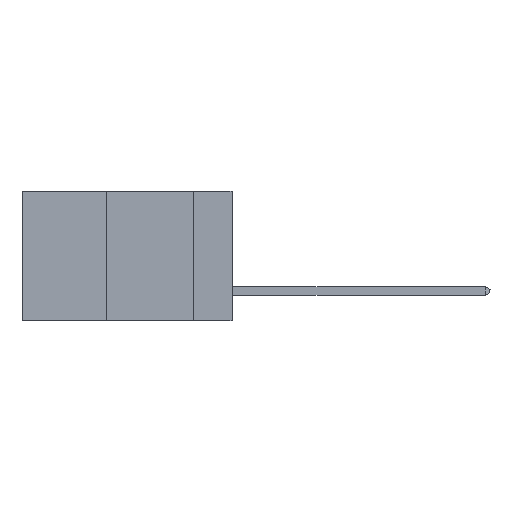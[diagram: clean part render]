
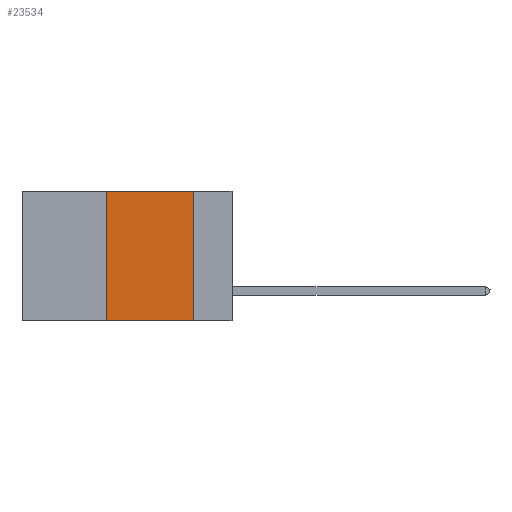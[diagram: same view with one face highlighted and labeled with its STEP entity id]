
A CAD part, left-side view. The second image highlights one B-rep face of the part: STEP entity #23534.
In plain terms, the highlighted planar face has unit normal (-1, 0, 0).
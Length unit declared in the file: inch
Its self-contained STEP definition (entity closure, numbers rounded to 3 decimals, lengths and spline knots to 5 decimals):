
#1942 = CARTESIAN_POINT ( 'NONE',  ( 0., 0.36, -0.37 ) ) ;
#3524 = LINE ( 'NONE', #8708, #16030 ) ;
#3607 = AXIS2_PLACEMENT_3D ( 'NONE', #24682, #27036, #29435 ) ;
#5075 = CARTESIAN_POINT ( 'NONE',  ( 0., 0.6, -0.37 ) ) ;
#5225 = EDGE_CURVE ( 'NONE', #8585, #28571, #3524, .T. ) ;
#8219 = EDGE_CURVE ( 'NONE', #16767, #28571, #21747, .T. ) ;
#8585 = VERTEX_POINT ( 'NONE', #18085 ) ;
#8708 = CARTESIAN_POINT ( 'NONE',  ( 0., 0.11, 0. ) ) ;
#9195 = VECTOR ( 'NONE', #16427, 39.37008 ) ;
#10290 = LINE ( 'NONE', #11520, #25818 ) ;
#11520 = CARTESIAN_POINT ( 'NONE',  ( 0., 0.6, 0. ) ) ;
#13164 = DIRECTION ( 'NONE',  ( 0., 0., -1. ) ) ;
#15195 = FACE_OUTER_BOUND ( 'NONE', #17914, .T. ) ;
#15750 = ORIENTED_EDGE ( 'NONE', *, *, #20838, .F. ) ;
#16030 = VECTOR ( 'NONE', #13164, 39.37008 ) ;
#16261 = LINE ( 'NONE', #18060, #23617 ) ;
#16427 = DIRECTION ( 'NONE',  ( 0., -1., 0. ) ) ;
#16767 = VERTEX_POINT ( 'NONE', #1942 ) ;
#17839 = ORIENTED_EDGE ( 'NONE', *, *, #8219, .T. ) ;
#17914 = EDGE_LOOP ( 'NONE', ( #25005, #18111, #15750, #17839 ) ) ;
#18060 = CARTESIAN_POINT ( 'NONE',  ( 0., 0.36, 0. ) ) ;
#18085 = CARTESIAN_POINT ( 'NONE',  ( 0., 0.11, 0. ) ) ;
#18111 = ORIENTED_EDGE ( 'NONE', *, *, #28934, .F. ) ;
#18945 = VERTEX_POINT ( 'NONE', #29068 ) ;
#19933 = PLANE ( 'NONE',  #3607 ) ;
#20731 = DIRECTION ( 'NONE',  ( 0., 0., 1. ) ) ;
#20838 = EDGE_CURVE ( 'NONE', #16767, #18945, #16261, .T. ) ;
#21747 = LINE ( 'NONE', #5075, #9195 ) ;
#23534 = ADVANCED_FACE ( 'NONE', ( #15195 ), #19933, .F. ) ;
#23617 = VECTOR ( 'NONE', #20731, 39.37008 ) ;
#24682 = CARTESIAN_POINT ( 'NONE',  ( 0., 0.6, 0. ) ) ;
#25005 = ORIENTED_EDGE ( 'NONE', *, *, #5225, .F. ) ;
#25770 = DIRECTION ( 'NONE',  ( 0., -1., 0. ) ) ;
#25818 = VECTOR ( 'NONE', #25770, 39.37008 ) ;
#27036 = DIRECTION ( 'NONE',  ( 1., 0., 0. ) ) ;
#28571 = VERTEX_POINT ( 'NONE', #29661 ) ;
#28934 = EDGE_CURVE ( 'NONE', #18945, #8585, #10290, .T. ) ;
#29068 = CARTESIAN_POINT ( 'NONE',  ( 0., 0.36, 0. ) ) ;
#29435 = DIRECTION ( 'NONE',  ( 0., 0., -1. ) ) ;
#29661 = CARTESIAN_POINT ( 'NONE',  ( 0., 0.11, -0.37 ) ) ;
